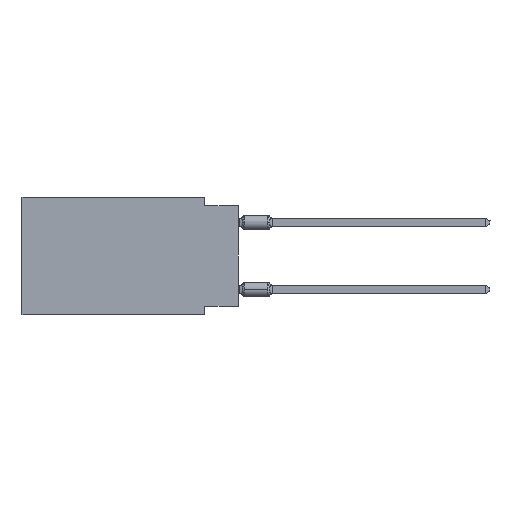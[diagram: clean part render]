
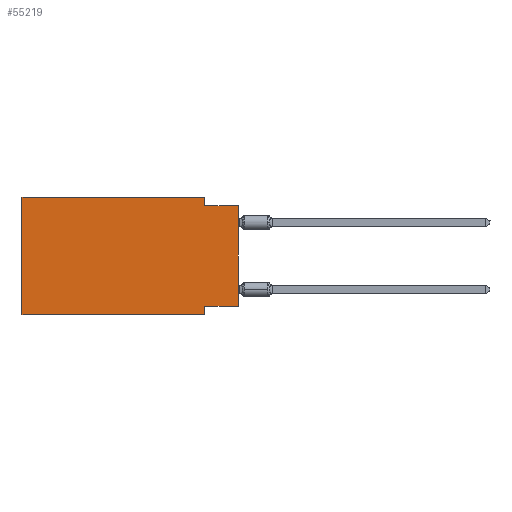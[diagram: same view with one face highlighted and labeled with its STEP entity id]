
A CAD part, left-side view. The second image highlights one B-rep face of the part: STEP entity #55219.
In plain terms, the highlighted planar face has unit normal (-1, 0, 0).
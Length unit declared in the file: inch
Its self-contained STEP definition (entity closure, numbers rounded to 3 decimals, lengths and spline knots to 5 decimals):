
#3861 = CARTESIAN_POINT ( 'NONE',  ( 0., 0.645, 0. ) ) ;
#4073 = CARTESIAN_POINT ( 'NONE',  ( 0., 0., -0.025 ) ) ;
#6245 = CARTESIAN_POINT ( 'NONE',  ( 0., 0.645, 0. ) ) ;
#7320 = ORIENTED_EDGE ( 'NONE', *, *, #37794, .T. ) ;
#7596 = CARTESIAN_POINT ( 'NONE',  ( 0., 0.1, -0.35 ) ) ;
#7680 = CARTESIAN_POINT ( 'NONE',  ( 0., 0.1, 0. ) ) ;
#7806 = LINE ( 'NONE', #30796, #34814 ) ;
#8838 = DIRECTION ( 'NONE',  ( 0., 1., 0. ) ) ;
#9905 = CARTESIAN_POINT ( 'NONE',  ( 0., 0., -0.325 ) ) ;
#10027 = CARTESIAN_POINT ( 'NONE',  ( 0., 0.645, -0.35 ) ) ;
#10523 = EDGE_LOOP ( 'NONE', ( #55995, #25362, #28979, #26897, #41912, #7320, #11705, #67116 ) ) ;
#11077 = CARTESIAN_POINT ( 'NONE',  ( 0., 0., 0. ) ) ;
#11259 = VERTEX_POINT ( 'NONE', #29759 ) ;
#11430 = EDGE_CURVE ( 'NONE', #40651, #11259, #36705, .T. ) ;
#11705 = ORIENTED_EDGE ( 'NONE', *, *, #43214, .F. ) ;
#14851 = VECTOR ( 'NONE', #54538, 39.37008 ) ;
#16099 = FACE_OUTER_BOUND ( 'NONE', #10523, .T. ) ;
#16454 = CARTESIAN_POINT ( 'NONE',  ( 0., 0.1, -0.025 ) ) ;
#16661 = VECTOR ( 'NONE', #42000, 39.37008 ) ;
#17113 = VERTEX_POINT ( 'NONE', #39094 ) ;
#19652 = EDGE_CURVE ( 'NONE', #11259, #23975, #31467, .T. ) ;
#23975 = VERTEX_POINT ( 'NONE', #7680 ) ;
#23987 = CARTESIAN_POINT ( 'NONE',  ( 0., 0., -0.325 ) ) ;
#24419 = VERTEX_POINT ( 'NONE', #7596 ) ;
#24832 = EDGE_CURVE ( 'NONE', #39475, #17113, #66875, .T. ) ;
#25017 = VECTOR ( 'NONE', #50796, 39.37008 ) ;
#25074 = EDGE_CURVE ( 'NONE', #39475, #46861, #31095, .T. ) ;
#25362 = ORIENTED_EDGE ( 'NONE', *, *, #50020, .F. ) ;
#26897 = ORIENTED_EDGE ( 'NONE', *, *, #19652, .F. ) ;
#28979 = ORIENTED_EDGE ( 'NONE', *, *, #48628, .F. ) ;
#29759 = CARTESIAN_POINT ( 'NONE',  ( 0., 0.645, 0. ) ) ;
#30597 = LINE ( 'NONE', #64507, #44528 ) ;
#30796 = CARTESIAN_POINT ( 'NONE',  ( 0., 0.1, -0.35 ) ) ;
#31095 = LINE ( 'NONE', #9905, #55290 ) ;
#31467 = LINE ( 'NONE', #6245, #63062 ) ;
#31567 = DIRECTION ( 'NONE',  ( 0., 0., 1. ) ) ;
#34586 = CARTESIAN_POINT ( 'NONE',  ( 0., 0.645, 0. ) ) ;
#34629 = CARTESIAN_POINT ( 'NONE',  ( 0., 0.645, -0.35 ) ) ;
#34814 = VECTOR ( 'NONE', #69452, 39.37008 ) ;
#36705 = LINE ( 'NONE', #3861, #56009 ) ;
#37794 = EDGE_CURVE ( 'NONE', #40651, #24419, #43248, .T. ) ;
#39094 = CARTESIAN_POINT ( 'NONE',  ( 0., 0., -0.025 ) ) ;
#39475 = VERTEX_POINT ( 'NONE', #23987 ) ;
#40651 = VERTEX_POINT ( 'NONE', #34629 ) ;
#41536 = DIRECTION ( 'NONE',  ( 0., 0., -1. ) ) ;
#41912 = ORIENTED_EDGE ( 'NONE', *, *, #11430, .F. ) ;
#42000 = DIRECTION ( 'NONE',  ( 0., -1., 0. ) ) ;
#43214 = EDGE_CURVE ( 'NONE', #46861, #24419, #7806, .T. ) ;
#43248 = LINE ( 'NONE', #10027, #14851 ) ;
#44528 = VECTOR ( 'NONE', #41536, 39.37008 ) ;
#46861 = VERTEX_POINT ( 'NONE', #69543 ) ;
#48628 = EDGE_CURVE ( 'NONE', #23975, #71343, #30597, .T. ) ;
#50020 = EDGE_CURVE ( 'NONE', #71343, #17113, #54021, .T. ) ;
#50796 = DIRECTION ( 'NONE',  ( 0., 0., 1. ) ) ;
#54021 = LINE ( 'NONE', #4073, #16661 ) ;
#54538 = DIRECTION ( 'NONE',  ( 0., -1., 0. ) ) ;
#55219 = ADVANCED_FACE ( 'NONE', ( #16099 ), #71892, .F. ) ;
#55290 = VECTOR ( 'NONE', #8838, 39.37008 ) ;
#55995 = ORIENTED_EDGE ( 'NONE', *, *, #24832, .T. ) ;
#56009 = VECTOR ( 'NONE', #31567, 39.37008 ) ;
#56819 = DIRECTION ( 'NONE',  ( 1., 0., 0. ) ) ;
#60247 = DIRECTION ( 'NONE',  ( 0., 0., -1. ) ) ;
#61519 = AXIS2_PLACEMENT_3D ( 'NONE', #34586, #56819, #60247 ) ;
#62045 = DIRECTION ( 'NONE',  ( 0., -1., 0. ) ) ;
#63062 = VECTOR ( 'NONE', #62045, 39.37008 ) ;
#64507 = CARTESIAN_POINT ( 'NONE',  ( 0., 0.1, 0. ) ) ;
#66875 = LINE ( 'NONE', #11077, #25017 ) ;
#67116 = ORIENTED_EDGE ( 'NONE', *, *, #25074, .F. ) ;
#69452 = DIRECTION ( 'NONE',  ( 0., 0., -1. ) ) ;
#69543 = CARTESIAN_POINT ( 'NONE',  ( 0., 0.1, -0.325 ) ) ;
#71343 = VERTEX_POINT ( 'NONE', #16454 ) ;
#71892 = PLANE ( 'NONE',  #61519 ) ;
